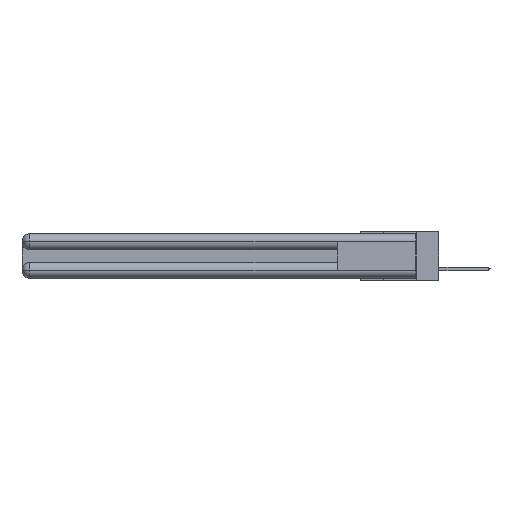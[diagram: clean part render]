
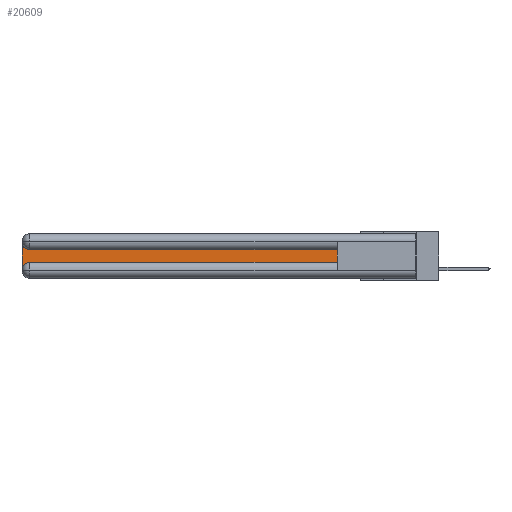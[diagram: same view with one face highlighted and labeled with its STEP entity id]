
A CAD part, left-side view. The second image highlights one B-rep face of the part: STEP entity #20609.
In plain terms, the highlighted planar face has unit normal (-1, 0, 0).
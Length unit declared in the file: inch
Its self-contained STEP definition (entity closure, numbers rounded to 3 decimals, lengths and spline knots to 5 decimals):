
#937 = ORIENTED_EDGE ( 'NONE', *, *, #1879, .T. ) ;
#1104 = DIRECTION ( 'NONE',  ( 1., 0., 0. ) ) ;
#1853 = CARTESIAN_POINT ( 'NONE',  ( 0.075, 0.6, -0.1225 ) ) ;
#1879 = EDGE_CURVE ( 'NONE', #24178, #15648, #22341, .T. ) ;
#2786 = VERTEX_POINT ( 'NONE', #13073 ) ;
#2796 = FACE_OUTER_BOUND ( 'NONE', #25982, .T. ) ;
#2824 = CARTESIAN_POINT ( 'NONE',  ( 0.075, 3., -0.2175 ) ) ;
#3726 = CARTESIAN_POINT ( 'NONE',  ( 0.075, 0.6, -0.2175 ) ) ;
#4052 = CARTESIAN_POINT ( 'NONE',  ( 0.075, 2.94, -0.2775 ) ) ;
#4269 = CARTESIAN_POINT ( 'NONE',  ( 0.075, 2.94, -0.0625 ) ) ;
#4937 = ORIENTED_EDGE ( 'NONE', *, *, #6363, .T. ) ;
#5162 = CARTESIAN_POINT ( 'NONE',  ( 0.075, 0.6, -0.2175 ) ) ;
#5870 = VERTEX_POINT ( 'NONE', #5162 ) ;
#6109 = CARTESIAN_POINT ( 'NONE',  ( 0.075, 0.6, -0.1225 ) ) ;
#6346 = DIRECTION ( 'NONE',  ( 1., 0., 0. ) ) ;
#6363 = EDGE_CURVE ( 'NONE', #16591, #24178, #29472, .T. ) ;
#7382 = LINE ( 'NONE', #16492, #9879 ) ;
#7805 = PLANE ( 'NONE',  #11782 ) ;
#8618 = DIRECTION ( 'NONE',  ( 0., -1., 0. ) ) ;
#8909 = VERTEX_POINT ( 'NONE', #11373 ) ;
#9815 = ORIENTED_EDGE ( 'NONE', *, *, #27354, .T. ) ;
#9870 = AXIS2_PLACEMENT_3D ( 'NONE', #4052, #6346, #20189 ) ;
#9879 = VECTOR ( 'NONE', #26313, 39.37008 ) ;
#9930 = LINE ( 'NONE', #2824, #21754 ) ;
#11373 = CARTESIAN_POINT ( 'NONE',  ( 0.075, 3., -0.2775 ) ) ;
#11551 = CARTESIAN_POINT ( 'NONE',  ( 0.075, 3., -0.0625 ) ) ;
#11782 = AXIS2_PLACEMENT_3D ( 'NONE', #28468, #1104, #23553 ) ;
#12122 = CIRCLE ( 'NONE', #9870, 0.06 ) ;
#13073 = CARTESIAN_POINT ( 'NONE',  ( 0.075, 2.94, -0.2175 ) ) ;
#15648 = VERTEX_POINT ( 'NONE', #11551 ) ;
#16492 = CARTESIAN_POINT ( 'NONE',  ( 0.075, 0.6, -0.2175 ) ) ;
#16532 = EDGE_CURVE ( 'NONE', #2786, #5870, #22935, .T. ) ;
#16591 = VERTEX_POINT ( 'NONE', #6109 ) ;
#18865 = DIRECTION ( 'NONE',  ( 0., 0., -1. ) ) ;
#19209 = ORIENTED_EDGE ( 'NONE', *, *, #20365, .T. ) ;
#19283 = ORIENTED_EDGE ( 'NONE', *, *, #16532, .T. ) ;
#20112 = VECTOR ( 'NONE', #8618, 39.37008 ) ;
#20189 = DIRECTION ( 'NONE',  ( 0., 0., -1. ) ) ;
#20365 = EDGE_CURVE ( 'NONE', #8909, #2786, #12122, .T. ) ;
#20609 = ADVANCED_FACE ( 'NONE', ( #2796 ), #7805, .F. ) ;
#21225 = CARTESIAN_POINT ( 'NONE',  ( 0.075, 2.94, -0.1225 ) ) ;
#21754 = VECTOR ( 'NONE', #18865, 39.37008 ) ;
#22341 = CIRCLE ( 'NONE', #28586, 0.06 ) ;
#22597 = DIRECTION ( 'NONE',  ( 1., 0., 0. ) ) ;
#22921 = ORIENTED_EDGE ( 'NONE', *, *, #26560, .T. ) ;
#22935 = LINE ( 'NONE', #3726, #20112 ) ;
#23553 = DIRECTION ( 'NONE',  ( 0., 0., -1. ) ) ;
#24178 = VERTEX_POINT ( 'NONE', #21225 ) ;
#25982 = EDGE_LOOP ( 'NONE', ( #4937, #937, #22921, #19209, #19283, #9815 ) ) ;
#26313 = DIRECTION ( 'NONE',  ( 0., 0., 1. ) ) ;
#26560 = EDGE_CURVE ( 'NONE', #15648, #8909, #9930, .T. ) ;
#27110 = DIRECTION ( 'NONE',  ( 0., 0., -1. ) ) ;
#27318 = VECTOR ( 'NONE', #29227, 39.37008 ) ;
#27354 = EDGE_CURVE ( 'NONE', #5870, #16591, #7382, .T. ) ;
#28468 = CARTESIAN_POINT ( 'NONE',  ( 0.075, 3., -0.1225 ) ) ;
#28586 = AXIS2_PLACEMENT_3D ( 'NONE', #4269, #22597, #27110 ) ;
#29227 = DIRECTION ( 'NONE',  ( 0., 1., 0. ) ) ;
#29472 = LINE ( 'NONE', #1853, #27318 ) ;
